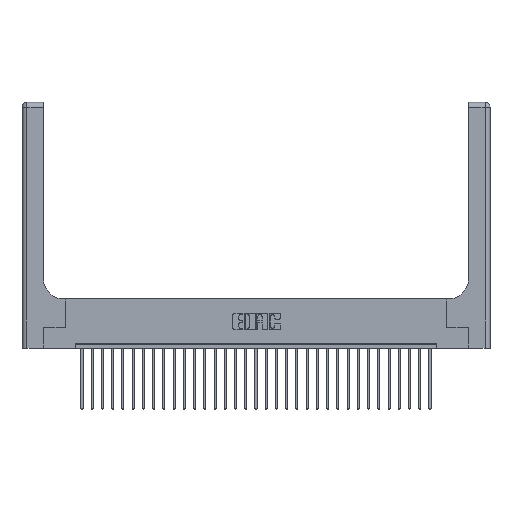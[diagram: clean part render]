
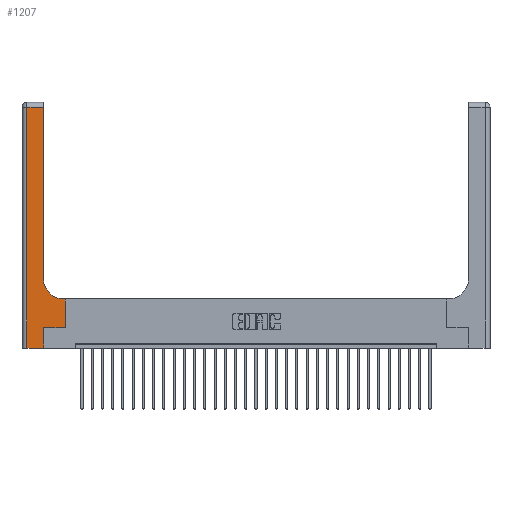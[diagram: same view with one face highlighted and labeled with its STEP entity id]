
A CAD part, top view. The second image highlights one B-rep face of the part: STEP entity #1207.
In plain terms, the highlighted planar face has unit normal (0, 0, 1).
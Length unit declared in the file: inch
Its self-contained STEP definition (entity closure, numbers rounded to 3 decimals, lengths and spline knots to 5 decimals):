
#55 = CARTESIAN_POINT ( 'NONE',  ( 0.51, 0.6, 0.37 ) ) ;
#202 = VECTOR ( 'NONE', #2432, 39.37008 ) ;
#217 = EDGE_CURVE ( 'NONE', #22930, #17435, #1992, .T. ) ;
#503 = VECTOR ( 'NONE', #2830, 39.37008 ) ;
#715 = VECTOR ( 'NONE', #23528, 39.37008 ) ;
#1207 = ADVANCED_FACE ( 'NONE', ( #4583 ), #26306, .F. ) ;
#1992 = LINE ( 'NONE', #10730, #7555 ) ;
#2432 = DIRECTION ( 'NONE',  ( 1., 0., 0. ) ) ;
#2830 = DIRECTION ( 'NONE',  ( 1., 0., 0. ) ) ;
#3356 = ORIENTED_EDGE ( 'NONE', *, *, #17444, .T. ) ;
#3507 = ORIENTED_EDGE ( 'NONE', *, *, #16988, .T. ) ;
#4200 = ORIENTED_EDGE ( 'NONE', *, *, #25125, .T. ) ;
#4583 = FACE_OUTER_BOUND ( 'NONE', #11893, .T. ) ;
#4740 = EDGE_CURVE ( 'NONE', #19090, #22930, #27574, .T. ) ;
#4835 = DIRECTION ( 'NONE',  ( 0., 0., -1. ) ) ;
#5067 = LINE ( 'NONE', #20338, #9993 ) ;
#5651 = AXIS2_PLACEMENT_3D ( 'NONE', #11671, #4835, #11256 ) ;
#7243 = DIRECTION ( 'NONE',  ( 0., 1., 0. ) ) ;
#7555 = VECTOR ( 'NONE', #28184, 39.37008 ) ;
#7618 = LINE ( 'NONE', #20615, #7830 ) ;
#7679 = CARTESIAN_POINT ( 'NONE',  ( 0.06, 0., 0.37 ) ) ;
#7830 = VECTOR ( 'NONE', #9753, 39.37008 ) ;
#9118 = VERTEX_POINT ( 'NONE', #20554 ) ;
#9478 = DIRECTION ( 'NONE',  ( 0., -1., 0. ) ) ;
#9644 = CARTESIAN_POINT ( 'NONE',  ( 0.26, 0.85, 0.37 ) ) ;
#9753 = DIRECTION ( 'NONE',  ( -1., 0., 0. ) ) ;
#9993 = VECTOR ( 'NONE', #9478, 39.37008 ) ;
#10730 = CARTESIAN_POINT ( 'NONE',  ( 0.26, 3., 0.37 ) ) ;
#11256 = DIRECTION ( 'NONE',  ( 1., 0., 0. ) ) ;
#11605 = VERTEX_POINT ( 'NONE', #24904 ) ;
#11671 = CARTESIAN_POINT ( 'NONE',  ( 0.51, 0.85, 0.37 ) ) ;
#11893 = EDGE_LOOP ( 'NONE', ( #13950, #15426, #18786, #4200, #15161, #3507, #3356, #19232, #18020 ) ) ;
#12512 = CARTESIAN_POINT ( 'NONE',  ( 0.528, 0.6, 0.37 ) ) ;
#13143 = EDGE_CURVE ( 'NONE', #18889, #19090, #7618, .T. ) ;
#13689 = DIRECTION ( 'NONE',  ( -1., 0., 0. ) ) ;
#13950 = ORIENTED_EDGE ( 'NONE', *, *, #217, .T. ) ;
#14370 = EDGE_CURVE ( 'NONE', #24585, #22515, #5067, .T. ) ;
#14544 = EDGE_CURVE ( 'NONE', #11605, #9118, #16885, .T. ) ;
#15161 = ORIENTED_EDGE ( 'NONE', *, *, #14544, .T. ) ;
#15426 = ORIENTED_EDGE ( 'NONE', *, *, #24668, .T. ) ;
#15548 = VERTEX_POINT ( 'NONE', #27861 ) ;
#15555 = DIRECTION ( 'NONE',  ( 0., 0., -1. ) ) ;
#15581 = LINE ( 'NONE', #22060, #202 ) ;
#15791 = CARTESIAN_POINT ( 'NONE',  ( 0.26, 2.94, 0.37 ) ) ;
#16885 = LINE ( 'NONE', #22789, #20046 ) ;
#16955 = VECTOR ( 'NONE', #7243, 39.37008 ) ;
#16988 = EDGE_CURVE ( 'NONE', #9118, #15548, #18262, .T. ) ;
#17435 = VERTEX_POINT ( 'NONE', #15791 ) ;
#17444 = EDGE_CURVE ( 'NONE', #15548, #18889, #18226, .T. ) ;
#18020 = ORIENTED_EDGE ( 'NONE', *, *, #4740, .T. ) ;
#18226 = LINE ( 'NONE', #22270, #16955 ) ;
#18262 = LINE ( 'NONE', #20695, #503 ) ;
#18463 = DIRECTION ( 'NONE',  ( 0., 1., 0. ) ) ;
#18786 = ORIENTED_EDGE ( 'NONE', *, *, #14370, .T. ) ;
#18889 = VERTEX_POINT ( 'NONE', #12512 ) ;
#19090 = VERTEX_POINT ( 'NONE', #55 ) ;
#19232 = ORIENTED_EDGE ( 'NONE', *, *, #13143, .T. ) ;
#19629 = LINE ( 'NONE', #21214, #715 ) ;
#20046 = VECTOR ( 'NONE', #18463, 39.37008 ) ;
#20338 = CARTESIAN_POINT ( 'NONE',  ( 0.06, 3., 0.37 ) ) ;
#20554 = CARTESIAN_POINT ( 'NONE',  ( 0.265, 0.25, 0.37 ) ) ;
#20615 = CARTESIAN_POINT ( 'NONE',  ( 0.26, 0.6, 0.37 ) ) ;
#20695 = CARTESIAN_POINT ( 'NONE',  ( 0.265, 0.25, 0.37 ) ) ;
#21214 = CARTESIAN_POINT ( 'NONE',  ( 0., 2.94, 0.37 ) ) ;
#21428 = AXIS2_PLACEMENT_3D ( 'NONE', #24170, #15555, #13689 ) ;
#22060 = CARTESIAN_POINT ( 'NONE',  ( 0., 0., 0.37 ) ) ;
#22270 = CARTESIAN_POINT ( 'NONE',  ( 0.528, 0.25, 0.37 ) ) ;
#22515 = VERTEX_POINT ( 'NONE', #7679 ) ;
#22789 = CARTESIAN_POINT ( 'NONE',  ( 0.265, 0., 0.37 ) ) ;
#22930 = VERTEX_POINT ( 'NONE', #9644 ) ;
#23528 = DIRECTION ( 'NONE',  ( -1., 0., 0. ) ) ;
#24170 = CARTESIAN_POINT ( 'NONE',  ( 0., 3., 0.37 ) ) ;
#24585 = VERTEX_POINT ( 'NONE', #25096 ) ;
#24668 = EDGE_CURVE ( 'NONE', #17435, #24585, #19629, .T. ) ;
#24904 = CARTESIAN_POINT ( 'NONE',  ( 0.265, 0., 0.37 ) ) ;
#25096 = CARTESIAN_POINT ( 'NONE',  ( 0.06, 2.94, 0.37 ) ) ;
#25125 = EDGE_CURVE ( 'NONE', #22515, #11605, #15581, .T. ) ;
#26306 = PLANE ( 'NONE',  #21428 ) ;
#27574 = CIRCLE ( 'NONE', #5651, 0.25 ) ;
#27861 = CARTESIAN_POINT ( 'NONE',  ( 0.528, 0.25, 0.37 ) ) ;
#28184 = DIRECTION ( 'NONE',  ( 0., 1., 0. ) ) ;
